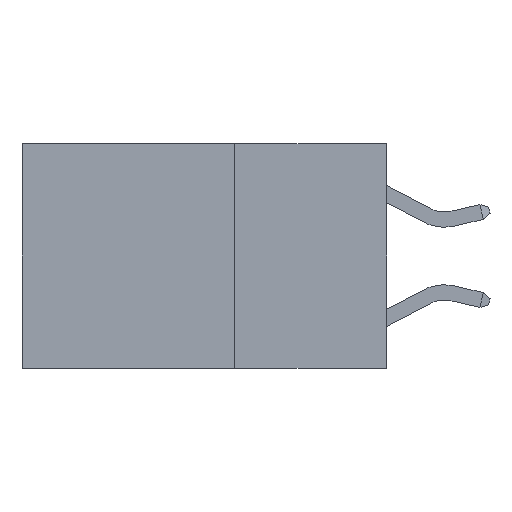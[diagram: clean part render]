
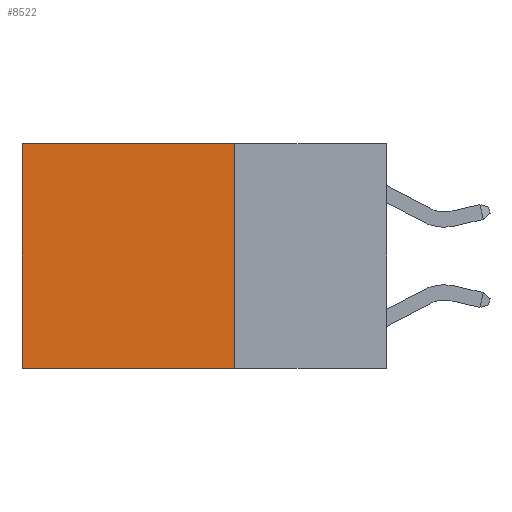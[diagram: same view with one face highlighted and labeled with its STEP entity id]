
A CAD part, left-side view. The second image highlights one B-rep face of the part: STEP entity #8522.
In plain terms, the highlighted planar face has unit normal (-1, 0, 0).
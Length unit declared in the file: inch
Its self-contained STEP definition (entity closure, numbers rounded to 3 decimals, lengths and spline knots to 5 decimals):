
#131 = LINE ( 'NONE', #10786, #2923 ) ;
#273 = ORIENTED_EDGE ( 'NONE', *, *, #3425, .F. ) ;
#469 = CARTESIAN_POINT ( 'NONE',  ( 0.2625, 0.6, 0. ) ) ;
#839 = LINE ( 'NONE', #9385, #4369 ) ;
#1239 = ORIENTED_EDGE ( 'NONE', *, *, #11009, .T. ) ;
#1532 = VECTOR ( 'NONE', #3562, 39.37008 ) ;
#2594 = ORIENTED_EDGE ( 'NONE', *, *, #6985, .F. ) ;
#2897 = AXIS2_PLACEMENT_3D ( 'NONE', #10990, #7846, #6757 ) ;
#2923 = VECTOR ( 'NONE', #6435, 39.37008 ) ;
#3278 = CARTESIAN_POINT ( 'NONE',  ( 0.2625, 0.6, 0. ) ) ;
#3399 = VECTOR ( 'NONE', #12563, 39.37008 ) ;
#3425 = EDGE_CURVE ( 'NONE', #6957, #13619, #131, .T. ) ;
#3562 = DIRECTION ( 'NONE',  ( 0., 1., 0. ) ) ;
#4369 = VECTOR ( 'NONE', #9712, 39.37008 ) ;
#4853 = EDGE_CURVE ( 'NONE', #6957, #7604, #839, .T. ) ;
#5771 = LINE ( 'NONE', #469, #3399 ) ;
#6103 = EDGE_LOOP ( 'NONE', ( #1239, #2594, #273, #7378 ) ) ;
#6435 = DIRECTION ( 'NONE',  ( 0., 0., -1. ) ) ;
#6688 = PLANE ( 'NONE',  #2897 ) ;
#6757 = DIRECTION ( 'NONE',  ( 0., 0., -1. ) ) ;
#6904 = CARTESIAN_POINT ( 'NONE',  ( 0.2625, 0.25, 0. ) ) ;
#6957 = VERTEX_POINT ( 'NONE', #6904 ) ;
#6985 = EDGE_CURVE ( 'NONE', #13619, #12832, #8818, .T. ) ;
#7378 = ORIENTED_EDGE ( 'NONE', *, *, #4853, .T. ) ;
#7604 = VERTEX_POINT ( 'NONE', #3278 ) ;
#7846 = DIRECTION ( 'NONE',  ( 1., 0., 0. ) ) ;
#8522 = ADVANCED_FACE ( 'NONE', ( #13112 ), #6688, .F. ) ;
#8818 = LINE ( 'NONE', #13110, #1532 ) ;
#8948 = CARTESIAN_POINT ( 'NONE',  ( 0.2625, 0.6, -0.37 ) ) ;
#9385 = CARTESIAN_POINT ( 'NONE',  ( 0.2625, 0.25, 0. ) ) ;
#9712 = DIRECTION ( 'NONE',  ( 0., 1., 0. ) ) ;
#10786 = CARTESIAN_POINT ( 'NONE',  ( 0.2625, 0.25, 0. ) ) ;
#10924 = CARTESIAN_POINT ( 'NONE',  ( 0.2625, 0.25, -0.37 ) ) ;
#10990 = CARTESIAN_POINT ( 'NONE',  ( 0.2625, 0.25, 0. ) ) ;
#11009 = EDGE_CURVE ( 'NONE', #7604, #12832, #5771, .T. ) ;
#12563 = DIRECTION ( 'NONE',  ( 0., 0., -1. ) ) ;
#12832 = VERTEX_POINT ( 'NONE', #8948 ) ;
#13110 = CARTESIAN_POINT ( 'NONE',  ( 0.2625, 0.25, -0.37 ) ) ;
#13112 = FACE_OUTER_BOUND ( 'NONE', #6103, .T. ) ;
#13619 = VERTEX_POINT ( 'NONE', #10924 ) ;
